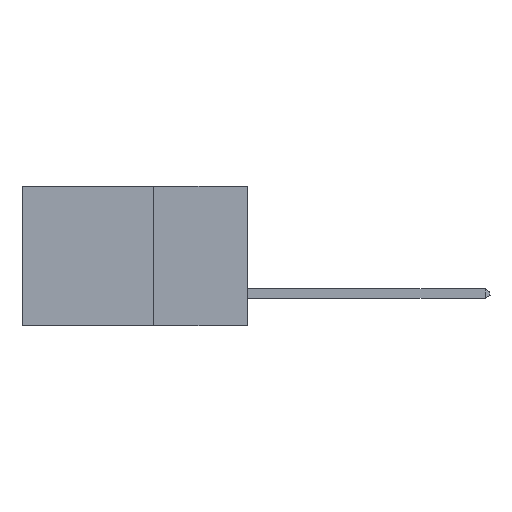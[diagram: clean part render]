
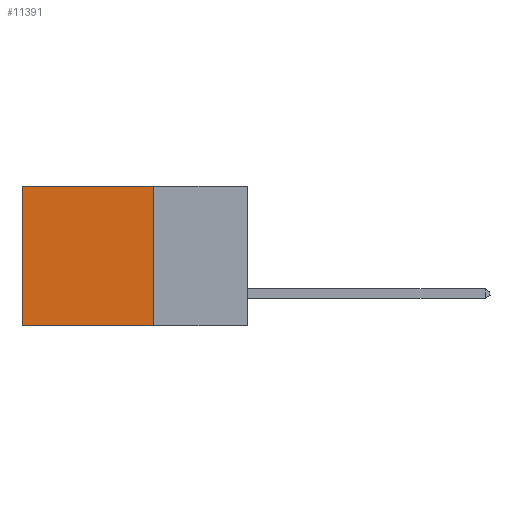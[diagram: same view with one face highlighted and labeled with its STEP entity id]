
A CAD part, left-side view. The second image highlights one B-rep face of the part: STEP entity #11391.
In plain terms, the highlighted planar face has unit normal (-1, 0, 0).
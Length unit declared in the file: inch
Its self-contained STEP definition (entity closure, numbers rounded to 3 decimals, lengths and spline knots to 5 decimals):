
#132 = EDGE_CURVE ( 'NONE', #4504, #15747, #10399, .T. ) ;
#514 = CARTESIAN_POINT ( 'NONE',  ( 0.298, 0.25, 0. ) ) ;
#820 = ORIENTED_EDGE ( 'NONE', *, *, #16245, .T. ) ;
#1266 = CARTESIAN_POINT ( 'NONE',  ( 0.298, 0.6, -0.37 ) ) ;
#1553 = VECTOR ( 'NONE', #16149, 39.37008 ) ;
#1846 = CARTESIAN_POINT ( 'NONE',  ( 0.298, 0.25, -0.37 ) ) ;
#2672 = EDGE_CURVE ( 'NONE', #4504, #11535, #8288, .T. ) ;
#4504 = VERTEX_POINT ( 'NONE', #10413 ) ;
#4744 = ORIENTED_EDGE ( 'NONE', *, *, #7050, .F. ) ;
#5249 = DIRECTION ( 'NONE',  ( 1., 0., 0. ) ) ;
#6037 = LINE ( 'NONE', #11495, #10062 ) ;
#6793 = EDGE_LOOP ( 'NONE', ( #820, #4744, #13610, #8794 ) ) ;
#7050 = EDGE_CURVE ( 'NONE', #15747, #13959, #13536, .T. ) ;
#7981 = AXIS2_PLACEMENT_3D ( 'NONE', #11532, #5249, #15549 ) ;
#8288 = LINE ( 'NONE', #10414, #14509 ) ;
#8794 = ORIENTED_EDGE ( 'NONE', *, *, #2672, .T. ) ;
#9589 = DIRECTION ( 'NONE',  ( 0., 0., -1. ) ) ;
#9783 = CARTESIAN_POINT ( 'NONE',  ( 0.298, 0.25, -0.37 ) ) ;
#10062 = VECTOR ( 'NONE', #15239, 39.37008 ) ;
#10399 = LINE ( 'NONE', #514, #15591 ) ;
#10413 = CARTESIAN_POINT ( 'NONE',  ( 0.298, 0.25, 0. ) ) ;
#10414 = CARTESIAN_POINT ( 'NONE',  ( 0.298, 0.25, 0. ) ) ;
#11391 = ADVANCED_FACE ( 'NONE', ( #15854 ), #12876, .F. ) ;
#11495 = CARTESIAN_POINT ( 'NONE',  ( 0.298, 0.6, 0. ) ) ;
#11532 = CARTESIAN_POINT ( 'NONE',  ( 0.298, 0.25, 0. ) ) ;
#11535 = VERTEX_POINT ( 'NONE', #12479 ) ;
#12479 = CARTESIAN_POINT ( 'NONE',  ( 0.298, 0.6, 0. ) ) ;
#12876 = PLANE ( 'NONE',  #7981 ) ;
#13042 = DIRECTION ( 'NONE',  ( 0., 1., 0. ) ) ;
#13536 = LINE ( 'NONE', #9783, #1553 ) ;
#13610 = ORIENTED_EDGE ( 'NONE', *, *, #132, .F. ) ;
#13959 = VERTEX_POINT ( 'NONE', #1266 ) ;
#14509 = VECTOR ( 'NONE', #13042, 39.37008 ) ;
#15239 = DIRECTION ( 'NONE',  ( 0., 0., -1. ) ) ;
#15549 = DIRECTION ( 'NONE',  ( 0., 0., -1. ) ) ;
#15591 = VECTOR ( 'NONE', #9589, 39.37008 ) ;
#15747 = VERTEX_POINT ( 'NONE', #1846 ) ;
#15854 = FACE_OUTER_BOUND ( 'NONE', #6793, .T. ) ;
#16149 = DIRECTION ( 'NONE',  ( 0., 1., 0. ) ) ;
#16245 = EDGE_CURVE ( 'NONE', #11535, #13959, #6037, .T. ) ;
